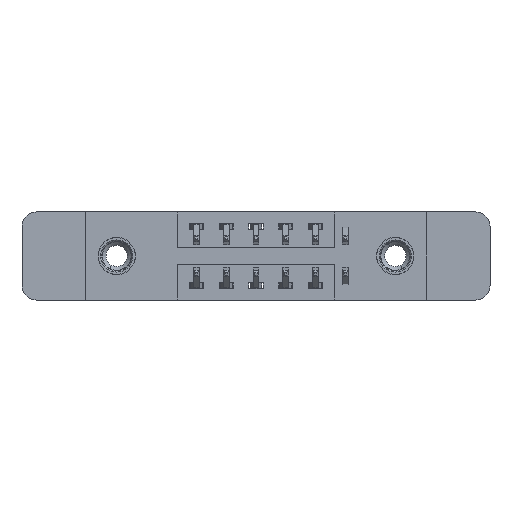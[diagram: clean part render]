
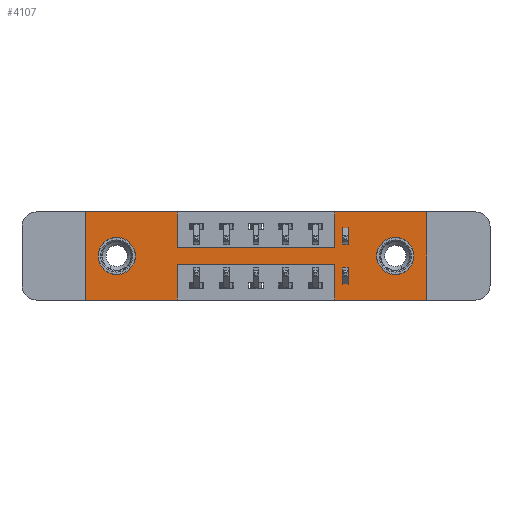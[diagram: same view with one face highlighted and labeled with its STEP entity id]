
A CAD part, front view. The second image highlights one B-rep face of the part: STEP entity #4107.
In plain terms, the highlighted planar face has unit normal (0, -1, 0).
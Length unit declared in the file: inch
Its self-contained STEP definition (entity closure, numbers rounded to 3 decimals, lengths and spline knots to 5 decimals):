
#60 = CIRCLE ( 'NONE', #12863, 0.078 ) ;
#290 = EDGE_CURVE ( 'NONE', #1674, #4853, #13339, .T. ) ;
#304 = CARTESIAN_POINT ( 'NONE',  ( 1.3025, 0., -0.107 ) ) ;
#431 = AXIS2_PLACEMENT_3D ( 'NONE', #9717, #3108, #9497 ) ;
#578 = CARTESIAN_POINT ( 'NONE',  ( 0., 0., -0.37 ) ) ;
#806 = ORIENTED_EDGE ( 'NONE', *, *, #892, .F. ) ;
#830 = LINE ( 'NONE', #1957, #7461 ) ;
#892 = EDGE_CURVE ( 'NONE', #7905, #4192, #13394, .T. ) ;
#975 = CARTESIAN_POINT ( 'NONE',  ( 0.3875, 0., -0.15 ) ) ;
#1097 = DIRECTION ( 'NONE',  ( 1., 0., 0. ) ) ;
#1104 = EDGE_CURVE ( 'NONE', #12672, #4122, #7718, .T. ) ;
#1383 = ORIENTED_EDGE ( 'NONE', *, *, #6070, .F. ) ;
#1457 = PLANE ( 'NONE',  #3116 ) ;
#1464 = VERTEX_POINT ( 'NONE', #7625 ) ;
#1626 = CARTESIAN_POINT ( 'NONE',  ( 1.0475, 0., 0. ) ) ;
#1674 = VERTEX_POINT ( 'NONE', #3737 ) ;
#1694 = LINE ( 'NONE', #2748, #1810 ) ;
#1747 = DIRECTION ( 'NONE',  ( 0., 0., -1. ) ) ;
#1784 = CARTESIAN_POINT ( 'NONE',  ( 0.1325, 0., -0.107 ) ) ;
#1810 = VECTOR ( 'NONE', #10366, 39.37008 ) ;
#1830 = CIRCLE ( 'NONE', #7298, 0.078 ) ;
#1878 = ORIENTED_EDGE ( 'NONE', *, *, #12995, .T. ) ;
#1883 = VECTOR ( 'NONE', #5733, 39.37008 ) ;
#1957 = CARTESIAN_POINT ( 'NONE',  ( 0.3875, 0., -0.22 ) ) ;
#2049 = CIRCLE ( 'NONE', #7772, 0.078 ) ;
#2153 = LINE ( 'NONE', #5149, #8073 ) ;
#2202 = LINE ( 'NONE', #3118, #2470 ) ;
#2253 = LINE ( 'NONE', #11004, #5475 ) ;
#2261 = CARTESIAN_POINT ( 'NONE',  ( 0., 0., 0. ) ) ;
#2470 = VECTOR ( 'NONE', #12946, 39.37008 ) ;
#2513 = DIRECTION ( 'NONE',  ( 0., -1., 0. ) ) ;
#2644 = FACE_BOUND ( 'NONE', #9209, .T. ) ;
#2748 = CARTESIAN_POINT ( 'NONE',  ( 0.3875, 0., -0.37 ) ) ;
#2895 = DIRECTION ( 'NONE',  ( 0., 0., 1. ) ) ;
#3028 = EDGE_CURVE ( 'NONE', #7785, #7602, #830, .T. ) ;
#3108 = DIRECTION ( 'NONE',  ( 0., 1., 0. ) ) ;
#3116 = AXIS2_PLACEMENT_3D ( 'NONE', #7963, #2513, #3591 ) ;
#3118 = CARTESIAN_POINT ( 'NONE',  ( 1.0475, 0., 0. ) ) ;
#3124 = ORIENTED_EDGE ( 'NONE', *, *, #1104, .F. ) ;
#3181 = ORIENTED_EDGE ( 'NONE', *, *, #12329, .T. ) ;
#3271 = ORIENTED_EDGE ( 'NONE', *, *, #10381, .F. ) ;
#3591 = DIRECTION ( 'NONE',  ( 0., 0., -1. ) ) ;
#3737 = CARTESIAN_POINT ( 'NONE',  ( 0.3875, 0., 0. ) ) ;
#3821 = CARTESIAN_POINT ( 'NONE',  ( 0.3875, 0., -0.15 ) ) ;
#3899 = ORIENTED_EDGE ( 'NONE', *, *, #9102, .F. ) ;
#3986 = CARTESIAN_POINT ( 'NONE',  ( 1.0475, 0., -0.22 ) ) ;
#4098 = LINE ( 'NONE', #975, #10975 ) ;
#4107 = ADVANCED_FACE ( 'NONE', ( #2644, #4790, #8091 ), #1457, .T. ) ;
#4122 = VERTEX_POINT ( 'NONE', #4859 ) ;
#4139 = VECTOR ( 'NONE', #6372, 39.37008 ) ;
#4191 = ORIENTED_EDGE ( 'NONE', *, *, #6459, .F. ) ;
#4192 = VERTEX_POINT ( 'NONE', #9040 ) ;
#4659 = EDGE_CURVE ( 'NONE', #4922, #7038, #2202, .T. ) ;
#4790 = FACE_BOUND ( 'NONE', #12080, .T. ) ;
#4847 = DIRECTION ( 'NONE',  ( 0., 0., -1. ) ) ;
#4853 = VERTEX_POINT ( 'NONE', #3821 ) ;
#4859 = CARTESIAN_POINT ( 'NONE',  ( 0., 0., 0. ) ) ;
#4922 = VERTEX_POINT ( 'NONE', #12253 ) ;
#5149 = CARTESIAN_POINT ( 'NONE',  ( 0., 0., 0. ) ) ;
#5212 = CIRCLE ( 'NONE', #431, 0.078 ) ;
#5398 = VERTEX_POINT ( 'NONE', #13040 ) ;
#5428 = CARTESIAN_POINT ( 'NONE',  ( 0., 0., -0.37 ) ) ;
#5475 = VECTOR ( 'NONE', #5552, 39.37008 ) ;
#5552 = DIRECTION ( 'NONE',  ( -1., 0., 0. ) ) ;
#5733 = DIRECTION ( 'NONE',  ( 0., 0., -1. ) ) ;
#5998 = CARTESIAN_POINT ( 'NONE',  ( 1.435, 0., 0. ) ) ;
#6070 = EDGE_CURVE ( 'NONE', #7602, #5398, #1694, .T. ) ;
#6273 = EDGE_CURVE ( 'NONE', #5398, #12672, #2253, .T. ) ;
#6281 = VERTEX_POINT ( 'NONE', #10726 ) ;
#6370 = ORIENTED_EDGE ( 'NONE', *, *, #7939, .T. ) ;
#6372 = DIRECTION ( 'NONE',  ( 1., 0., 0. ) ) ;
#6410 = ORIENTED_EDGE ( 'NONE', *, *, #13058, .F. ) ;
#6442 = CARTESIAN_POINT ( 'NONE',  ( 1.435, 0., 0. ) ) ;
#6459 = EDGE_CURVE ( 'NONE', #4853, #4922, #4098, .T. ) ;
#6625 = DIRECTION ( 'NONE',  ( 0., 0., 1. ) ) ;
#6765 = VERTEX_POINT ( 'NONE', #1784 ) ;
#6811 = CARTESIAN_POINT ( 'NONE',  ( 0.3875, 0., 0. ) ) ;
#7038 = VERTEX_POINT ( 'NONE', #1626 ) ;
#7070 = LINE ( 'NONE', #5998, #7878 ) ;
#7114 = DIRECTION ( 'NONE',  ( 0., 1., 0. ) ) ;
#7176 = DIRECTION ( 'NONE',  ( 0., 1., 0. ) ) ;
#7298 = AXIS2_PLACEMENT_3D ( 'NONE', #8486, #7114, #2895 ) ;
#7429 = ORIENTED_EDGE ( 'NONE', *, *, #3028, .F. ) ;
#7461 = VECTOR ( 'NONE', #7464, 39.37008 ) ;
#7464 = DIRECTION ( 'NONE',  ( -1., 0., 0. ) ) ;
#7491 = ORIENTED_EDGE ( 'NONE', *, *, #4659, .F. ) ;
#7538 = ORIENTED_EDGE ( 'NONE', *, *, #6273, .F. ) ;
#7602 = VERTEX_POINT ( 'NONE', #7807 ) ;
#7625 = CARTESIAN_POINT ( 'NONE',  ( 1.3025, 0., -0.263 ) ) ;
#7710 = CARTESIAN_POINT ( 'NONE',  ( 1.0475, 0., -0.37 ) ) ;
#7718 = LINE ( 'NONE', #2261, #8800 ) ;
#7772 = AXIS2_PLACEMENT_3D ( 'NONE', #14098, #12074, #11018 ) ;
#7785 = VERTEX_POINT ( 'NONE', #3986 ) ;
#7807 = CARTESIAN_POINT ( 'NONE',  ( 0.3875, 0., -0.22 ) ) ;
#7878 = VECTOR ( 'NONE', #4847, 39.37008 ) ;
#7905 = VERTEX_POINT ( 'NONE', #9446 ) ;
#7939 = EDGE_CURVE ( 'NONE', #9218, #1464, #2049, .T. ) ;
#7963 = CARTESIAN_POINT ( 'NONE',  ( 0., 0., -0.37 ) ) ;
#8073 = VECTOR ( 'NONE', #1097, 39.37008 ) ;
#8091 = FACE_OUTER_BOUND ( 'NONE', #9885, .T. ) ;
#8208 = EDGE_CURVE ( 'NONE', #6281, #6765, #1830, .T. ) ;
#8486 = CARTESIAN_POINT ( 'NONE',  ( 0.1325, 0., -0.185 ) ) ;
#8800 = VECTOR ( 'NONE', #6625, 39.37008 ) ;
#8822 = ORIENTED_EDGE ( 'NONE', *, *, #290, .F. ) ;
#9040 = CARTESIAN_POINT ( 'NONE',  ( 1.0475, 0., -0.37 ) ) ;
#9056 = VECTOR ( 'NONE', #9936, 39.37008 ) ;
#9102 = EDGE_CURVE ( 'NONE', #4122, #1674, #2153, .T. ) ;
#9155 = DIRECTION ( 'NONE',  ( -1., 0., 0. ) ) ;
#9209 = EDGE_LOOP ( 'NONE', ( #6370, #3181 ) ) ;
#9218 = VERTEX_POINT ( 'NONE', #304 ) ;
#9446 = CARTESIAN_POINT ( 'NONE',  ( 1.435, 0., -0.37 ) ) ;
#9497 = DIRECTION ( 'NONE',  ( 0., 0., 1. ) ) ;
#9630 = DIRECTION ( 'NONE',  ( 1., 0., 0. ) ) ;
#9717 = CARTESIAN_POINT ( 'NONE',  ( 0.1325, 0., -0.185 ) ) ;
#9885 = EDGE_LOOP ( 'NONE', ( #1383, #7429, #6410, #806, #3271, #13957, #7491, #4191, #8822, #3899, #3124, #7538 ) ) ;
#9936 = DIRECTION ( 'NONE',  ( 0., 0., 1. ) ) ;
#10366 = DIRECTION ( 'NONE',  ( 0., 0., -1. ) ) ;
#10381 = EDGE_CURVE ( 'NONE', #14002, #7905, #7070, .T. ) ;
#10396 = VECTOR ( 'NONE', #9155, 39.37008 ) ;
#10697 = LINE ( 'NONE', #11469, #4139 ) ;
#10726 = CARTESIAN_POINT ( 'NONE',  ( 0.1325, 0., -0.263 ) ) ;
#10868 = LINE ( 'NONE', #7710, #9056 ) ;
#10975 = VECTOR ( 'NONE', #9630, 39.37008 ) ;
#11004 = CARTESIAN_POINT ( 'NONE',  ( 0., 0., -0.37 ) ) ;
#11018 = DIRECTION ( 'NONE',  ( 0., 0., -1. ) ) ;
#11243 = ORIENTED_EDGE ( 'NONE', *, *, #8208, .T. ) ;
#11469 = CARTESIAN_POINT ( 'NONE',  ( 0., 0., 0. ) ) ;
#11766 = CARTESIAN_POINT ( 'NONE',  ( 1.3025, 0., -0.185 ) ) ;
#12074 = DIRECTION ( 'NONE',  ( 0., 1., 0. ) ) ;
#12080 = EDGE_LOOP ( 'NONE', ( #1878, #11243 ) ) ;
#12253 = CARTESIAN_POINT ( 'NONE',  ( 1.0475, 0., -0.15 ) ) ;
#12329 = EDGE_CURVE ( 'NONE', #1464, #9218, #60, .T. ) ;
#12672 = VERTEX_POINT ( 'NONE', #5428 ) ;
#12863 = AXIS2_PLACEMENT_3D ( 'NONE', #11766, #7176, #1747 ) ;
#12946 = DIRECTION ( 'NONE',  ( 0., 0., 1. ) ) ;
#12995 = EDGE_CURVE ( 'NONE', #6765, #6281, #5212, .T. ) ;
#13040 = CARTESIAN_POINT ( 'NONE',  ( 0.3875, 0., -0.37 ) ) ;
#13058 = EDGE_CURVE ( 'NONE', #4192, #7785, #10868, .T. ) ;
#13339 = LINE ( 'NONE', #6811, #1883 ) ;
#13394 = LINE ( 'NONE', #578, #10396 ) ;
#13946 = EDGE_CURVE ( 'NONE', #7038, #14002, #10697, .T. ) ;
#13957 = ORIENTED_EDGE ( 'NONE', *, *, #13946, .F. ) ;
#14002 = VERTEX_POINT ( 'NONE', #6442 ) ;
#14098 = CARTESIAN_POINT ( 'NONE',  ( 1.3025, 0., -0.185 ) ) ;
